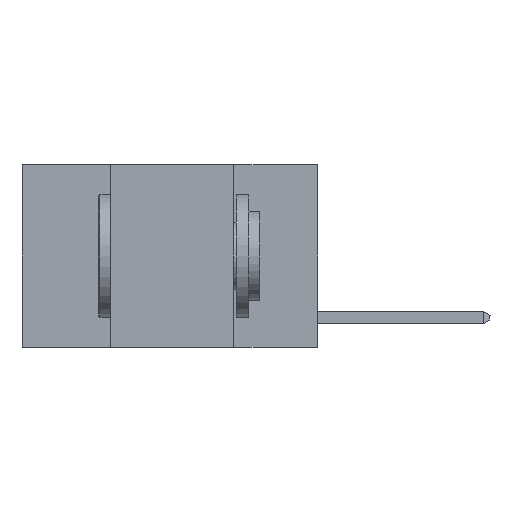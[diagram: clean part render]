
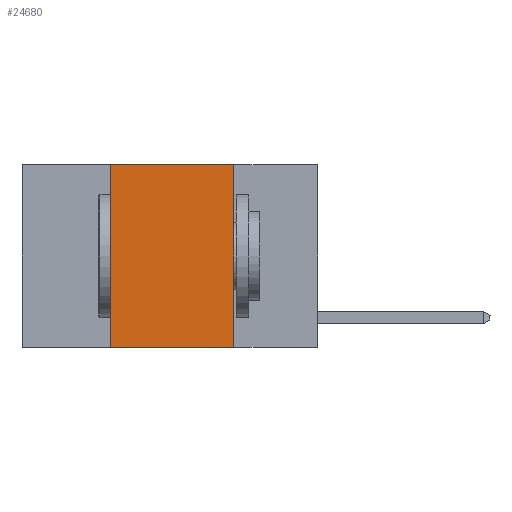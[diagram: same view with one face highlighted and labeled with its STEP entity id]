
A CAD part, left-side view. The second image highlights one B-rep face of the part: STEP entity #24680.
In plain terms, the highlighted planar face has unit normal (-1, 0, 0).
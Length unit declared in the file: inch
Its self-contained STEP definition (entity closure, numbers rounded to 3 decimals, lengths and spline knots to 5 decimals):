
#8 = CARTESIAN_POINT ( 'NONE',  ( 0., 0.17, 0. ) ) ;
#31 = CARTESIAN_POINT ( 'NONE',  ( 0., 0.6, 0. ) ) ;
#413 = AXIS2_PLACEMENT_3D ( 'NONE', #9114, #18581, #25247 ) ;
#2428 = EDGE_LOOP ( 'NONE', ( #29553, #23031, #5442, #27461 ) ) ;
#2890 = CARTESIAN_POINT ( 'NONE',  ( 0., 0.17, -0.37 ) ) ;
#2906 = EDGE_CURVE ( 'NONE', #28630, #25008, #16516, .T. ) ;
#3295 = DIRECTION ( 'NONE',  ( 0., 0., 1. ) ) ;
#5442 = ORIENTED_EDGE ( 'NONE', *, *, #10681, .F. ) ;
#6873 = DIRECTION ( 'NONE',  ( 0., -1., 0. ) ) ;
#7248 = CARTESIAN_POINT ( 'NONE',  ( 0., 0.17, 0. ) ) ;
#7567 = EDGE_CURVE ( 'NONE', #25008, #21659, #19207, .T. ) ;
#8104 = LINE ( 'NONE', #29378, #11342 ) ;
#9114 = CARTESIAN_POINT ( 'NONE',  ( 0., 0.6, 0. ) ) ;
#9872 = CARTESIAN_POINT ( 'NONE',  ( 0., 0.42, 0. ) ) ;
#10681 = EDGE_CURVE ( 'NONE', #11770, #28630, #8104, .T. ) ;
#11342 = VECTOR ( 'NONE', #3295, 39.37008 ) ;
#11770 = VERTEX_POINT ( 'NONE', #23503 ) ;
#13846 = EDGE_CURVE ( 'NONE', #11770, #21659, #28099, .T. ) ;
#14270 = VECTOR ( 'NONE', #26624, 39.37008 ) ;
#15806 = FACE_OUTER_BOUND ( 'NONE', #2428, .T. ) ;
#16182 = DIRECTION ( 'NONE',  ( 0., -1., 0. ) ) ;
#16412 = VECTOR ( 'NONE', #16182, 39.37008 ) ;
#16516 = LINE ( 'NONE', #31, #20881 ) ;
#18581 = DIRECTION ( 'NONE',  ( 1., 0., 0. ) ) ;
#19207 = LINE ( 'NONE', #7248, #14270 ) ;
#20881 = VECTOR ( 'NONE', #6873, 39.37008 ) ;
#21659 = VERTEX_POINT ( 'NONE', #2890 ) ;
#23031 = ORIENTED_EDGE ( 'NONE', *, *, #2906, .F. ) ;
#23503 = CARTESIAN_POINT ( 'NONE',  ( 0., 0.42, -0.37 ) ) ;
#24680 = ADVANCED_FACE ( 'NONE', ( #15806 ), #30380, .F. ) ;
#25008 = VERTEX_POINT ( 'NONE', #8 ) ;
#25247 = DIRECTION ( 'NONE',  ( 0., 0., -1. ) ) ;
#26624 = DIRECTION ( 'NONE',  ( 0., 0., -1. ) ) ;
#27461 = ORIENTED_EDGE ( 'NONE', *, *, #13846, .T. ) ;
#28099 = LINE ( 'NONE', #28410, #16412 ) ;
#28410 = CARTESIAN_POINT ( 'NONE',  ( 0., 0.6, -0.37 ) ) ;
#28630 = VERTEX_POINT ( 'NONE', #9872 ) ;
#29378 = CARTESIAN_POINT ( 'NONE',  ( 0., 0.42, 0. ) ) ;
#29553 = ORIENTED_EDGE ( 'NONE', *, *, #7567, .F. ) ;
#30380 = PLANE ( 'NONE',  #413 ) ;
